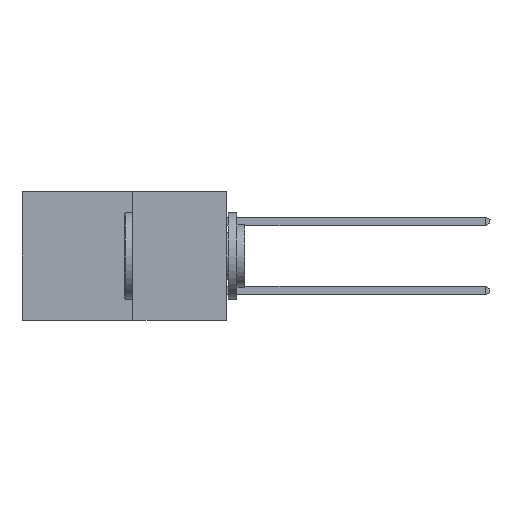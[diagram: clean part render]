
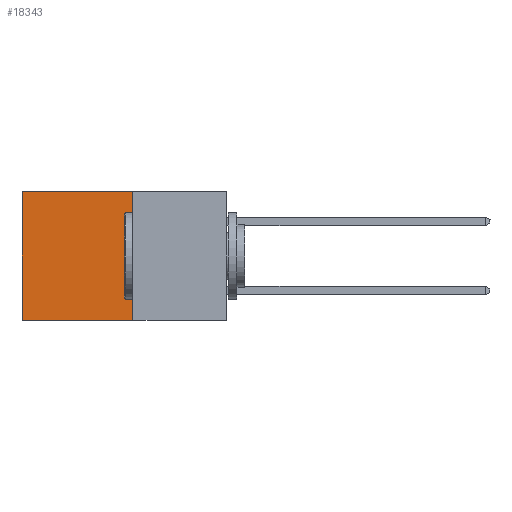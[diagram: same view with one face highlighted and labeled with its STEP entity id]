
A CAD part, left-side view. The second image highlights one B-rep face of the part: STEP entity #18343.
In plain terms, the highlighted planar face has unit normal (-1, 0, 0).
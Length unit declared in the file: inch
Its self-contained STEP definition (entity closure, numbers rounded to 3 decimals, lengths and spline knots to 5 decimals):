
#634 = CARTESIAN_POINT ( 'NONE',  ( 0.277, 0.59, -0.37 ) ) ;
#770 = VERTEX_POINT ( 'NONE', #13691 ) ;
#885 = CARTESIAN_POINT ( 'NONE',  ( 0.277, 0.27, 0. ) ) ;
#1288 = VERTEX_POINT ( 'NONE', #12000 ) ;
#3167 = VECTOR ( 'NONE', #3781, 39.37008 ) ;
#3781 = DIRECTION ( 'NONE',  ( 0., 1., 0. ) ) ;
#4238 = CARTESIAN_POINT ( 'NONE',  ( 0.277, 0.27, -0.37 ) ) ;
#4603 = VERTEX_POINT ( 'NONE', #7147 ) ;
#6013 = DIRECTION ( 'NONE',  ( 0., 1., 0. ) ) ;
#6256 = VECTOR ( 'NONE', #6013, 39.37008 ) ;
#6743 = LINE ( 'NONE', #885, #6256 ) ;
#7090 = CARTESIAN_POINT ( 'NONE',  ( 0.277, 0.27, -0.37 ) ) ;
#7132 = DIRECTION ( 'NONE',  ( 0., 0., -1. ) ) ;
#7147 = CARTESIAN_POINT ( 'NONE',  ( 0.277, 0.27, -0.37 ) ) ;
#7189 = EDGE_CURVE ( 'NONE', #4603, #10925, #11218, .T. ) ;
#7510 = VECTOR ( 'NONE', #7132, 39.37008 ) ;
#9112 = LINE ( 'NONE', #14549, #12491 ) ;
#10370 = AXIS2_PLACEMENT_3D ( 'NONE', #13776, #17397, #11780 ) ;
#10925 = VERTEX_POINT ( 'NONE', #634 ) ;
#11218 = LINE ( 'NONE', #4238, #3167 ) ;
#11346 = EDGE_CURVE ( 'NONE', #770, #1288, #6743, .T. ) ;
#11543 = PLANE ( 'NONE',  #10370 ) ;
#11780 = DIRECTION ( 'NONE',  ( 0., 0., -1. ) ) ;
#12000 = CARTESIAN_POINT ( 'NONE',  ( 0.277, 0.59, 0. ) ) ;
#12491 = VECTOR ( 'NONE', #14279, 39.37008 ) ;
#13691 = CARTESIAN_POINT ( 'NONE',  ( 0.277, 0.27, 0. ) ) ;
#13776 = CARTESIAN_POINT ( 'NONE',  ( 0.277, 0.27, -0.37 ) ) ;
#14279 = DIRECTION ( 'NONE',  ( 0., 0., -1. ) ) ;
#14549 = CARTESIAN_POINT ( 'NONE',  ( 0.277, 0.59, -0.37 ) ) ;
#14746 = LINE ( 'NONE', #7090, #7510 ) ;
#15579 = FACE_OUTER_BOUND ( 'NONE', #17815, .T. ) ;
#15691 = ORIENTED_EDGE ( 'NONE', *, *, #17531, .T. ) ;
#16519 = EDGE_CURVE ( 'NONE', #770, #4603, #14746, .T. ) ;
#17397 = DIRECTION ( 'NONE',  ( 1., 0., 0. ) ) ;
#17531 = EDGE_CURVE ( 'NONE', #1288, #10925, #9112, .T. ) ;
#17815 = EDGE_LOOP ( 'NONE', ( #15691, #18501, #19123, #18551 ) ) ;
#18343 = ADVANCED_FACE ( 'NONE', ( #15579 ), #11543, .F. ) ;
#18501 = ORIENTED_EDGE ( 'NONE', *, *, #7189, .F. ) ;
#18551 = ORIENTED_EDGE ( 'NONE', *, *, #11346, .T. ) ;
#19123 = ORIENTED_EDGE ( 'NONE', *, *, #16519, .F. ) ;
